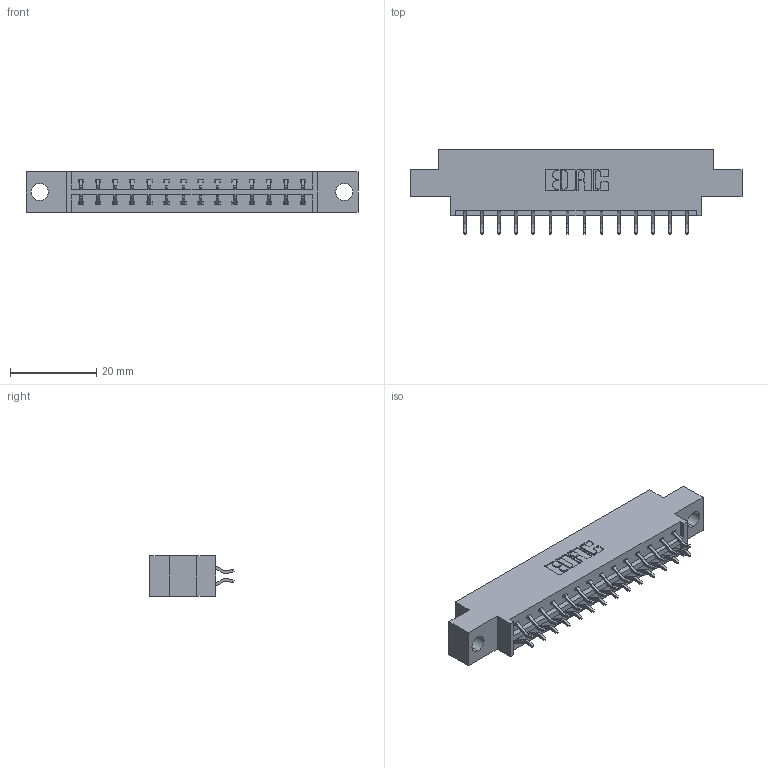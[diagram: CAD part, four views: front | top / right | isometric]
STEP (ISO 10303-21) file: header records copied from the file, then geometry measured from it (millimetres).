
FILE_DESCRIPTION (( 'STEP AP203' ), '1' );
FILE_NAME ('833-028-556-804.STEP', '2020-06-02T09:39:48', ( '' ), ( '' ), 'SwSTEP 2.0', 'SolidWorks 2020', '' );
FILE_SCHEMA (( 'CONFIG_CONTROL_DESIGN' ));
Length unit declared in the file: inch
Products named in the file (3): 345-292-001_556 Tail; 833 Part_Offset - .156 Dia - TH; 833-028-556-804
Assembly tree (29 placements, depth 2):
  833-028-556-804
    833 Part_Offset - .156 Dia - TH
    345-292-001_556 Tail  x28
Bounding box: 77.01 x 19.57 x 9.4 mm (x, y, z)
Volume: 7284 mm3; surface area: 8303.2 mm2
Topology: 29 solids, 29 shells, 1742 faces, 5167 edges, 3406 vertices
Faces by surface type: plane 1194, cylinder 548
Entity records: 12983 total; most frequent: CARTESIAN_POINT 2202, ORIENTED_EDGE 2126, DIRECTION 1919, EDGE_CURVE 1063, VECTOR 927, LINE 927, VERTEX_POINT 706, AXIS2_PLACEMENT_3D 496
